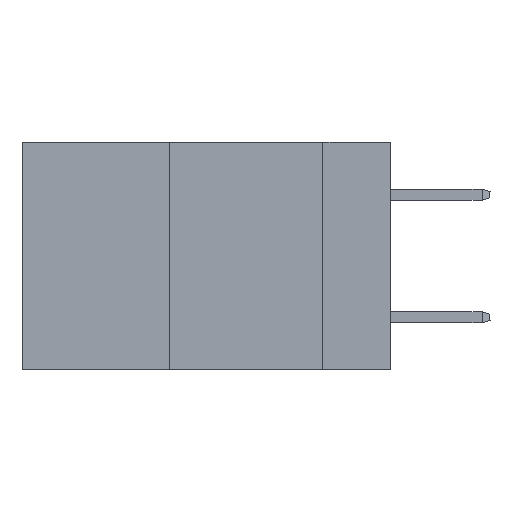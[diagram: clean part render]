
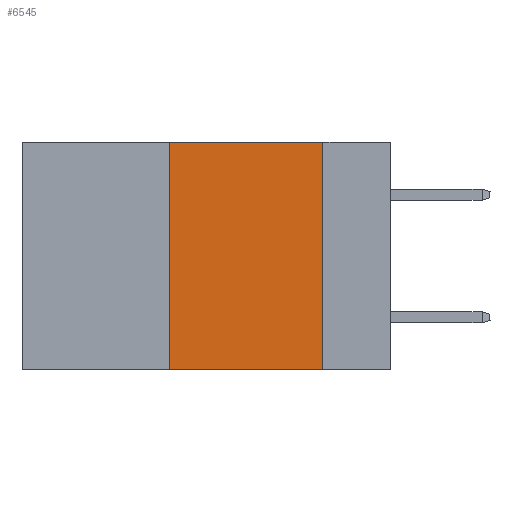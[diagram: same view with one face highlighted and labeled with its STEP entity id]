
A CAD part, left-side view. The second image highlights one B-rep face of the part: STEP entity #6545.
In plain terms, the highlighted planar face has unit normal (-1, 0, 0).
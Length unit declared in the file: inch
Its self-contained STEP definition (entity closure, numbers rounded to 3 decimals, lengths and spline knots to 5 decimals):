
#212 = ORIENTED_EDGE ( 'NONE', *, *, #17491, .F. ) ;
#1309 = CARTESIAN_POINT ( 'NONE',  ( 0., 0.6, 0. ) ) ;
#1593 = CARTESIAN_POINT ( 'NONE',  ( 0., 0.6, 0. ) ) ;
#1748 = VERTEX_POINT ( 'NONE', #14686 ) ;
#1810 = LINE ( 'NONE', #1309, #9818 ) ;
#2176 = FACE_OUTER_BOUND ( 'NONE', #7053, .T. ) ;
#2372 = CARTESIAN_POINT ( 'NONE',  ( 0., 0.11, 0. ) ) ;
#2635 = LINE ( 'NONE', #9984, #15122 ) ;
#3211 = DIRECTION ( 'NONE',  ( 0., 0., -1. ) ) ;
#3265 = VERTEX_POINT ( 'NONE', #19225 ) ;
#4369 = EDGE_CURVE ( 'NONE', #12904, #15225, #4556, .T. ) ;
#4495 = DIRECTION ( 'NONE',  ( 0., -1., 0. ) ) ;
#4556 = LINE ( 'NONE', #14009, #12428 ) ;
#6545 = ADVANCED_FACE ( 'NONE', ( #2176 ), #9598, .F. ) ;
#7053 = EDGE_LOOP ( 'NONE', ( #17642, #11406, #212, #16466 ) ) ;
#7955 = EDGE_CURVE ( 'NONE', #1748, #15225, #2635, .T. ) ;
#9168 = EDGE_CURVE ( 'NONE', #3265, #12904, #1810, .T. ) ;
#9364 = LINE ( 'NONE', #13053, #13431 ) ;
#9598 = PLANE ( 'NONE',  #10485 ) ;
#9818 = VECTOR ( 'NONE', #4495, 39.37008 ) ;
#9937 = DIRECTION ( 'NONE',  ( 0., 0., 1. ) ) ;
#9984 = CARTESIAN_POINT ( 'NONE',  ( 0., 0.6, -0.37 ) ) ;
#10485 = AXIS2_PLACEMENT_3D ( 'NONE', #1593, #12688, #3211 ) ;
#11406 = ORIENTED_EDGE ( 'NONE', *, *, #9168, .F. ) ;
#12428 = VECTOR ( 'NONE', #18730, 39.37008 ) ;
#12688 = DIRECTION ( 'NONE',  ( 1., 0., 0. ) ) ;
#12904 = VERTEX_POINT ( 'NONE', #2372 ) ;
#13053 = CARTESIAN_POINT ( 'NONE',  ( 0., 0.36, 0. ) ) ;
#13431 = VECTOR ( 'NONE', #9937, 39.37008 ) ;
#14009 = CARTESIAN_POINT ( 'NONE',  ( 0., 0.11, 0. ) ) ;
#14489 = DIRECTION ( 'NONE',  ( 0., -1., 0. ) ) ;
#14686 = CARTESIAN_POINT ( 'NONE',  ( 0., 0.36, -0.37 ) ) ;
#15122 = VECTOR ( 'NONE', #14489, 39.37008 ) ;
#15225 = VERTEX_POINT ( 'NONE', #18867 ) ;
#16466 = ORIENTED_EDGE ( 'NONE', *, *, #7955, .T. ) ;
#17491 = EDGE_CURVE ( 'NONE', #1748, #3265, #9364, .T. ) ;
#17642 = ORIENTED_EDGE ( 'NONE', *, *, #4369, .F. ) ;
#18730 = DIRECTION ( 'NONE',  ( 0., 0., -1. ) ) ;
#18867 = CARTESIAN_POINT ( 'NONE',  ( 0., 0.11, -0.37 ) ) ;
#19225 = CARTESIAN_POINT ( 'NONE',  ( 0., 0.36, 0. ) ) ;
